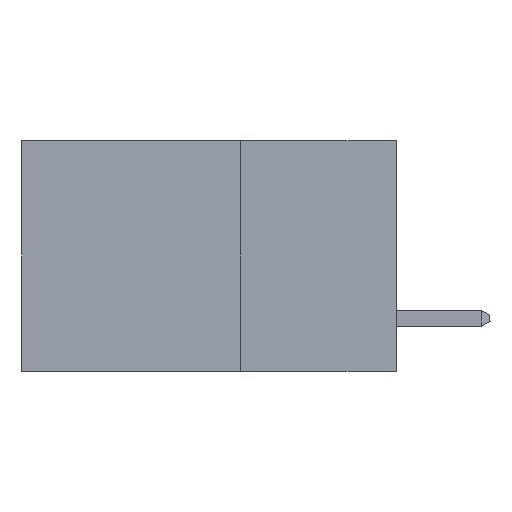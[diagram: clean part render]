
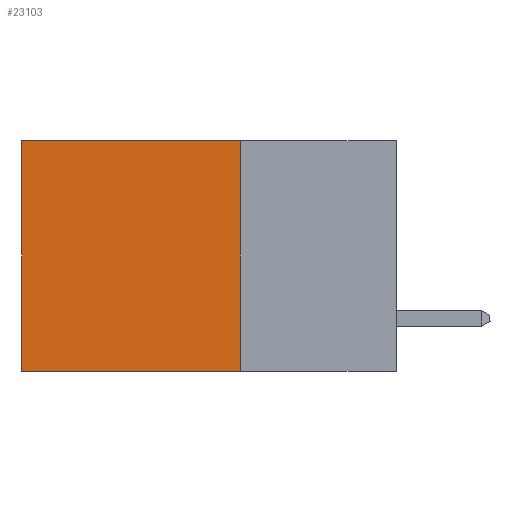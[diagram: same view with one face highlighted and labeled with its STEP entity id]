
A CAD part, left-side view. The second image highlights one B-rep face of the part: STEP entity #23103.
In plain terms, the highlighted planar face has unit normal (-1, 0, 0).
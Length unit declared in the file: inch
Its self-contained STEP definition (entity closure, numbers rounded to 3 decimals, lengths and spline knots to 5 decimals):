
#236 = ORIENTED_EDGE ( 'NONE', *, *, #21410, .F. ) ;
#2862 = EDGE_LOOP ( 'NONE', ( #15010, #22557, #236, #12071 ) ) ;
#2997 = AXIS2_PLACEMENT_3D ( 'NONE', #27388, #12521, #12415 ) ;
#3019 = LINE ( 'NONE', #21102, #20317 ) ;
#3379 = VERTEX_POINT ( 'NONE', #23764 ) ;
#3730 = VERTEX_POINT ( 'NONE', #27596 ) ;
#6195 = CARTESIAN_POINT ( 'NONE',  ( 0.298, 0.25, -0.37 ) ) ;
#9870 = VECTOR ( 'NONE', #27453, 39.37008 ) ;
#9879 = PLANE ( 'NONE',  #2997 ) ;
#10994 = DIRECTION ( 'NONE',  ( 0., 1., 0. ) ) ;
#11462 = VERTEX_POINT ( 'NONE', #12597 ) ;
#12071 = ORIENTED_EDGE ( 'NONE', *, *, #31415, .T. ) ;
#12415 = DIRECTION ( 'NONE',  ( 0., 0., -1. ) ) ;
#12521 = DIRECTION ( 'NONE',  ( 1., 0., 0. ) ) ;
#12545 = VECTOR ( 'NONE', #10994, 39.37008 ) ;
#12597 = CARTESIAN_POINT ( 'NONE',  ( 0.298, 0.6, -0.37 ) ) ;
#13386 = LINE ( 'NONE', #32371, #9870 ) ;
#14670 = EDGE_CURVE ( 'NONE', #3379, #11462, #3019, .T. ) ;
#14830 = FACE_OUTER_BOUND ( 'NONE', #2862, .T. ) ;
#15010 = ORIENTED_EDGE ( 'NONE', *, *, #14670, .T. ) ;
#16416 = LINE ( 'NONE', #20375, #17226 ) ;
#17226 = VECTOR ( 'NONE', #28526, 39.37008 ) ;
#20016 = LINE ( 'NONE', #30776, #12545 ) ;
#20317 = VECTOR ( 'NONE', #23808, 39.37008 ) ;
#20375 = CARTESIAN_POINT ( 'NONE',  ( 0.298, 0.25, 0. ) ) ;
#21102 = CARTESIAN_POINT ( 'NONE',  ( 0.298, 0.6, 0. ) ) ;
#21410 = EDGE_CURVE ( 'NONE', #3730, #31493, #13386, .T. ) ;
#22557 = ORIENTED_EDGE ( 'NONE', *, *, #29741, .F. ) ;
#23103 = ADVANCED_FACE ( 'NONE', ( #14830 ), #9879, .F. ) ;
#23764 = CARTESIAN_POINT ( 'NONE',  ( 0.298, 0.6, 0. ) ) ;
#23808 = DIRECTION ( 'NONE',  ( 0., 0., -1. ) ) ;
#27388 = CARTESIAN_POINT ( 'NONE',  ( 0.298, 0.25, 0. ) ) ;
#27453 = DIRECTION ( 'NONE',  ( 0., 0., -1. ) ) ;
#27596 = CARTESIAN_POINT ( 'NONE',  ( 0.298, 0.25, 0. ) ) ;
#28526 = DIRECTION ( 'NONE',  ( 0., 1., 0. ) ) ;
#29741 = EDGE_CURVE ( 'NONE', #31493, #11462, #20016, .T. ) ;
#30776 = CARTESIAN_POINT ( 'NONE',  ( 0.298, 0.25, -0.37 ) ) ;
#31415 = EDGE_CURVE ( 'NONE', #3730, #3379, #16416, .T. ) ;
#31493 = VERTEX_POINT ( 'NONE', #6195 ) ;
#32371 = CARTESIAN_POINT ( 'NONE',  ( 0.298, 0.25, 0. ) ) ;
